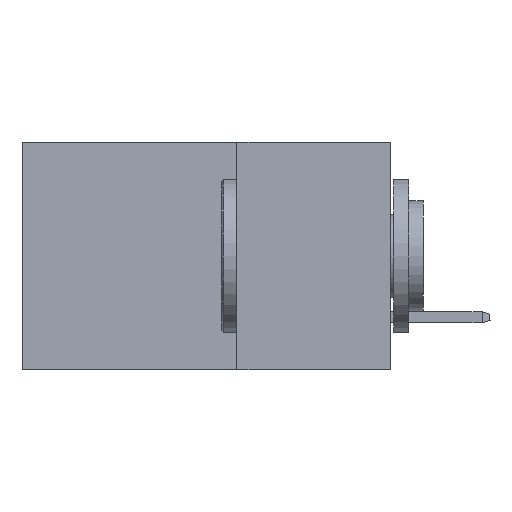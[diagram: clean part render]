
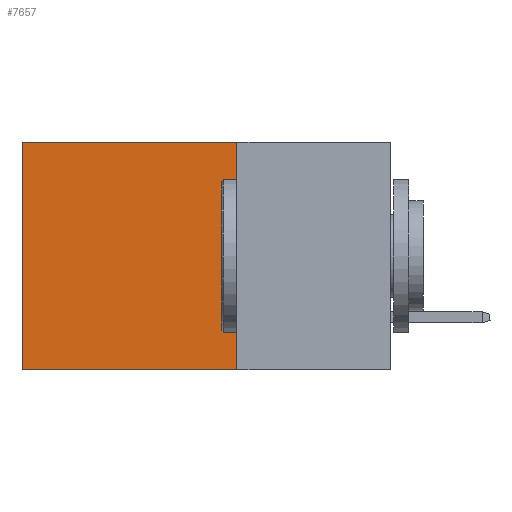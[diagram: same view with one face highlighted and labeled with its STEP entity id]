
A CAD part, left-side view. The second image highlights one B-rep face of the part: STEP entity #7657.
In plain terms, the highlighted planar face has unit normal (-1, 0, 0).
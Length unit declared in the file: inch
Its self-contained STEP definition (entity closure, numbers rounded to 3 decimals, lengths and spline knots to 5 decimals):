
#54 = ORIENTED_EDGE ( 'NONE', *, *, #7870, .T. ) ;
#880 = EDGE_CURVE ( 'NONE', #4525, #13056, #5958, .T. ) ;
#895 = AXIS2_PLACEMENT_3D ( 'NONE', #3517, #8155, #1229 ) ;
#1229 = DIRECTION ( 'NONE',  ( 0., 0., -1. ) ) ;
#1482 = ORIENTED_EDGE ( 'NONE', *, *, #7774, .F. ) ;
#2630 = DIRECTION ( 'NONE',  ( 0., 0., -1. ) ) ;
#3372 = CARTESIAN_POINT ( 'NONE',  ( 0.2875, 0.25, -0.37 ) ) ;
#3517 = CARTESIAN_POINT ( 'NONE',  ( 0.2875, 0.25, 0. ) ) ;
#3573 = ORIENTED_EDGE ( 'NONE', *, *, #880, .F. ) ;
#4439 = FACE_OUTER_BOUND ( 'NONE', #12361, .T. ) ;
#4525 = VERTEX_POINT ( 'NONE', #5448 ) ;
#4720 = VECTOR ( 'NONE', #5250, 39.37008 ) ;
#5250 = DIRECTION ( 'NONE',  ( 0., 1., 0. ) ) ;
#5448 = CARTESIAN_POINT ( 'NONE',  ( 0.2875, 0.25, 0. ) ) ;
#5834 = LINE ( 'NONE', #14547, #4720 ) ;
#5958 = LINE ( 'NONE', #10714, #7588 ) ;
#6028 = ORIENTED_EDGE ( 'NONE', *, *, #6620, .T. ) ;
#6212 = CARTESIAN_POINT ( 'NONE',  ( 0.2875, 0.6, 0. ) ) ;
#6620 = EDGE_CURVE ( 'NONE', #4525, #15046, #5834, .T. ) ;
#6984 = LINE ( 'NONE', #6212, #9652 ) ;
#7336 = VECTOR ( 'NONE', #13582, 39.37008 ) ;
#7588 = VECTOR ( 'NONE', #11951, 39.37008 ) ;
#7657 = ADVANCED_FACE ( 'NONE', ( #4439 ), #13818, .F. ) ;
#7774 = EDGE_CURVE ( 'NONE', #13056, #14890, #14427, .T. ) ;
#7870 = EDGE_CURVE ( 'NONE', #15046, #14890, #6984, .T. ) ;
#8155 = DIRECTION ( 'NONE',  ( 1., 0., 0. ) ) ;
#8552 = CARTESIAN_POINT ( 'NONE',  ( 0.2875, 0.6, -0.37 ) ) ;
#9652 = VECTOR ( 'NONE', #2630, 39.37008 ) ;
#10714 = CARTESIAN_POINT ( 'NONE',  ( 0.2875, 0.25, 0. ) ) ;
#11363 = CARTESIAN_POINT ( 'NONE',  ( 0.2875, 0.6, 0. ) ) ;
#11951 = DIRECTION ( 'NONE',  ( 0., 0., -1. ) ) ;
#12361 = EDGE_LOOP ( 'NONE', ( #54, #1482, #3573, #6028 ) ) ;
#13056 = VERTEX_POINT ( 'NONE', #3372 ) ;
#13195 = CARTESIAN_POINT ( 'NONE',  ( 0.2875, 0.25, -0.37 ) ) ;
#13582 = DIRECTION ( 'NONE',  ( 0., 1., 0. ) ) ;
#13818 = PLANE ( 'NONE',  #895 ) ;
#14427 = LINE ( 'NONE', #13195, #7336 ) ;
#14547 = CARTESIAN_POINT ( 'NONE',  ( 0.2875, 0.25, 0. ) ) ;
#14890 = VERTEX_POINT ( 'NONE', #8552 ) ;
#15046 = VERTEX_POINT ( 'NONE', #11363 ) ;
